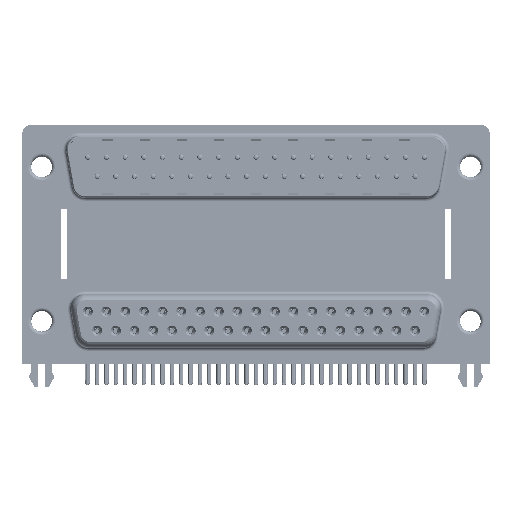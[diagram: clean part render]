
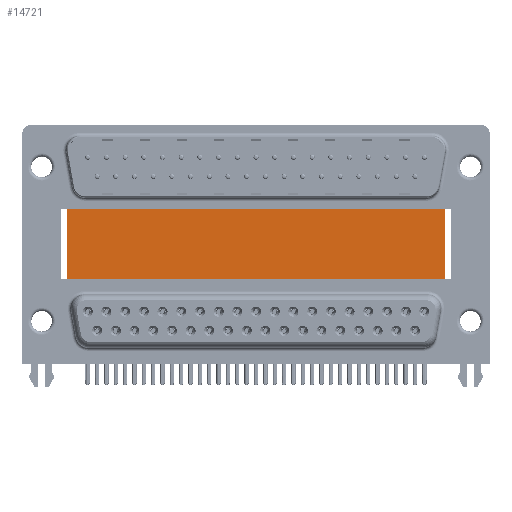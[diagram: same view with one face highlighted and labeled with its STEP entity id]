
A CAD part, top view. The second image highlights one B-rep face of the part: STEP entity #14721.
In plain terms, the highlighted planar face has unit normal (0, 0, 1).
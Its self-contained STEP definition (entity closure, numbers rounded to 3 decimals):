
#1849 = CARTESIAN_POINT ( 'NONE',  ( 59.71, 16.585, -12. ) ) ;
#3536 = DIRECTION ( 'NONE',  ( -1., 0., 0. ) ) ;
#4863 = LINE ( 'NONE', #47319, #29883 ) ;
#10963 = DIRECTION ( 'NONE',  ( 0., -1., 0. ) ) ;
#12014 = EDGE_CURVE ( 'NONE', #19728, #39015, #36829, .T. ) ;
#12243 = VERTEX_POINT ( 'NONE', #33066 ) ;
#13470 = LINE ( 'NONE', #34175, #46751 ) ;
#14721 = ADVANCED_FACE ( 'NONE', ( #29323 ), #66031, .F. ) ;
#19023 = EDGE_CURVE ( 'NONE', #55832, #39015, #4863, .T. ) ;
#19134 = EDGE_LOOP ( 'NONE', ( #40201, #22866, #39566, #53869 ) ) ;
#19728 = VERTEX_POINT ( 'NONE', #21945 ) ;
#21945 = CARTESIAN_POINT ( 'NONE',  ( 3.79, -3.735, -12. ) ) ;
#22866 = ORIENTED_EDGE ( 'NONE', *, *, #19023, .F. ) ;
#22867 = VECTOR ( 'NONE', #29509, 1000. ) ;
#22975 = CARTESIAN_POINT ( 'NONE',  ( 59.71, -3.735, -12. ) ) ;
#29323 = FACE_OUTER_BOUND ( 'NONE', #19134, .T. ) ;
#29509 = DIRECTION ( 'NONE',  ( 1., 0., 0. ) ) ;
#29883 = VECTOR ( 'NONE', #10963, 1000. ) ;
#33066 = CARTESIAN_POINT ( 'NONE',  ( 3.79, 16.585, -12. ) ) ;
#33604 = LINE ( 'NONE', #60105, #22867 ) ;
#34175 = CARTESIAN_POINT ( 'NONE',  ( 3.79, 16.585, -12. ) ) ;
#36829 = LINE ( 'NONE', #41592, #62502 ) ;
#37755 = EDGE_CURVE ( 'NONE', #12243, #19728, #13470, .T. ) ;
#38270 = DIRECTION ( 'NONE',  ( 0., -1., 0. ) ) ;
#38592 = EDGE_CURVE ( 'NONE', #12243, #55832, #33604, .T. ) ;
#39015 = VERTEX_POINT ( 'NONE', #22975 ) ;
#39566 = ORIENTED_EDGE ( 'NONE', *, *, #38592, .F. ) ;
#40201 = ORIENTED_EDGE ( 'NONE', *, *, #12014, .T. ) ;
#41592 = CARTESIAN_POINT ( 'NONE',  ( 3.79, -3.735, -12. ) ) ;
#44133 = AXIS2_PLACEMENT_3D ( 'NONE', #60250, #55838, #3536 ) ;
#46702 = DIRECTION ( 'NONE',  ( 1., 0., 0. ) ) ;
#46751 = VECTOR ( 'NONE', #38270, 1000. ) ;
#47319 = CARTESIAN_POINT ( 'NONE',  ( 59.71, 16.585, -12. ) ) ;
#53869 = ORIENTED_EDGE ( 'NONE', *, *, #37755, .T. ) ;
#55832 = VERTEX_POINT ( 'NONE', #1849 ) ;
#55838 = DIRECTION ( 'NONE',  ( 0., 0., -1. ) ) ;
#60105 = CARTESIAN_POINT ( 'NONE',  ( 3.79, 16.585, -12. ) ) ;
#60250 = CARTESIAN_POINT ( 'NONE',  ( 3.79, 16.585, -12. ) ) ;
#62502 = VECTOR ( 'NONE', #46702, 1000. ) ;
#66031 = PLANE ( 'NONE',  #44133 ) ;
